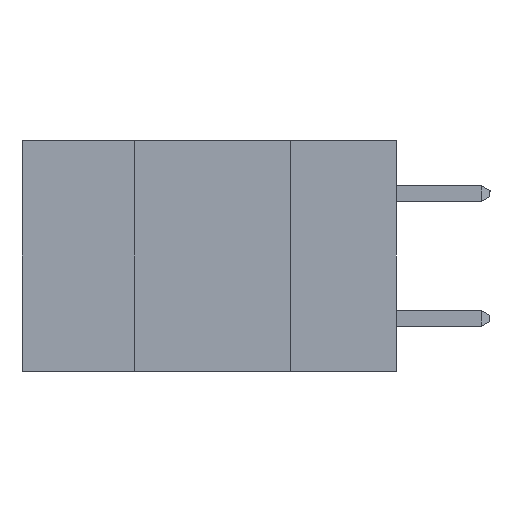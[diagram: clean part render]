
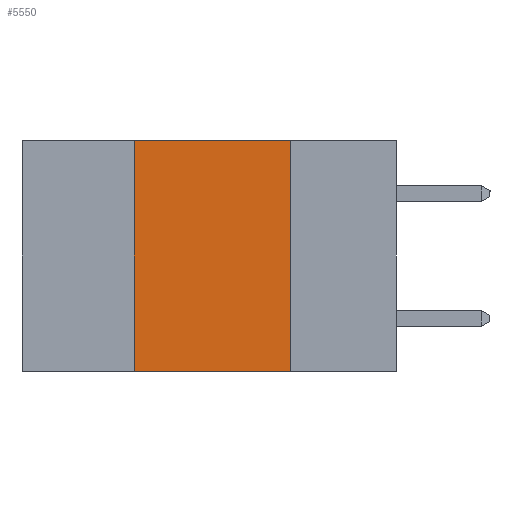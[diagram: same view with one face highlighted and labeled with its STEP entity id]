
A CAD part, left-side view. The second image highlights one B-rep face of the part: STEP entity #5550.
In plain terms, the highlighted planar face has unit normal (-1, 0, 0).
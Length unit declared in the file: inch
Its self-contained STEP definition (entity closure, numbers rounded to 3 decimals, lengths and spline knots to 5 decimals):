
#899 = VECTOR ( 'NONE', #16911, 39.37008 ) ;
#1287 = EDGE_LOOP ( 'NONE', ( #18471, #14520, #17095, #16449 ) ) ;
#1618 = CARTESIAN_POINT ( 'NONE',  ( 0., 0.6, 0. ) ) ;
#1840 = CARTESIAN_POINT ( 'NONE',  ( 0., 0.42, -0.37 ) ) ;
#1859 = LINE ( 'NONE', #4628, #8393 ) ;
#2092 = DIRECTION ( 'NONE',  ( 0., 0., -1. ) ) ;
#2302 = CARTESIAN_POINT ( 'NONE',  ( 0., 0.42, -0.37 ) ) ;
#2359 = VERTEX_POINT ( 'NONE', #4080 ) ;
#2955 = CARTESIAN_POINT ( 'NONE',  ( 0., 0.6, 0. ) ) ;
#3030 = DIRECTION ( 'NONE',  ( 0., 0., -1. ) ) ;
#3769 = EDGE_CURVE ( 'NONE', #15063, #2359, #6354, .T. ) ;
#4080 = CARTESIAN_POINT ( 'NONE',  ( 0., 0.42, 0. ) ) ;
#4310 = DIRECTION ( 'NONE',  ( 0., -1., 0. ) ) ;
#4628 = CARTESIAN_POINT ( 'NONE',  ( 0., 0.17, -0.37 ) ) ;
#5266 = AXIS2_PLACEMENT_3D ( 'NONE', #1618, #6139, #2092 ) ;
#5550 = ADVANCED_FACE ( 'NONE', ( #6052 ), #15123, .F. ) ;
#5889 = LINE ( 'NONE', #7363, #6000 ) ;
#6000 = VECTOR ( 'NONE', #4310, 39.37008 ) ;
#6052 = FACE_OUTER_BOUND ( 'NONE', #1287, .T. ) ;
#6139 = DIRECTION ( 'NONE',  ( 1., 0., 0. ) ) ;
#6190 = VECTOR ( 'NONE', #16306, 39.37008 ) ;
#6354 = LINE ( 'NONE', #2302, #899 ) ;
#6919 = CARTESIAN_POINT ( 'NONE',  ( 0., 0.17, -0.37 ) ) ;
#7363 = CARTESIAN_POINT ( 'NONE',  ( 0., 0.6, -0.37 ) ) ;
#8393 = VECTOR ( 'NONE', #3030, 39.37008 ) ;
#11057 = EDGE_CURVE ( 'NONE', #14558, #12483, #1859, .T. ) ;
#11728 = EDGE_CURVE ( 'NONE', #2359, #14558, #19454, .T. ) ;
#12483 = VERTEX_POINT ( 'NONE', #6919 ) ;
#12594 = CARTESIAN_POINT ( 'NONE',  ( 0., 0.17, 0. ) ) ;
#14520 = ORIENTED_EDGE ( 'NONE', *, *, #11728, .F. ) ;
#14558 = VERTEX_POINT ( 'NONE', #12594 ) ;
#15063 = VERTEX_POINT ( 'NONE', #1840 ) ;
#15123 = PLANE ( 'NONE',  #5266 ) ;
#16306 = DIRECTION ( 'NONE',  ( 0., -1., 0. ) ) ;
#16449 = ORIENTED_EDGE ( 'NONE', *, *, #18221, .T. ) ;
#16911 = DIRECTION ( 'NONE',  ( 0., 0., 1. ) ) ;
#17095 = ORIENTED_EDGE ( 'NONE', *, *, #3769, .F. ) ;
#18221 = EDGE_CURVE ( 'NONE', #15063, #12483, #5889, .T. ) ;
#18471 = ORIENTED_EDGE ( 'NONE', *, *, #11057, .F. ) ;
#19454 = LINE ( 'NONE', #2955, #6190 ) ;
